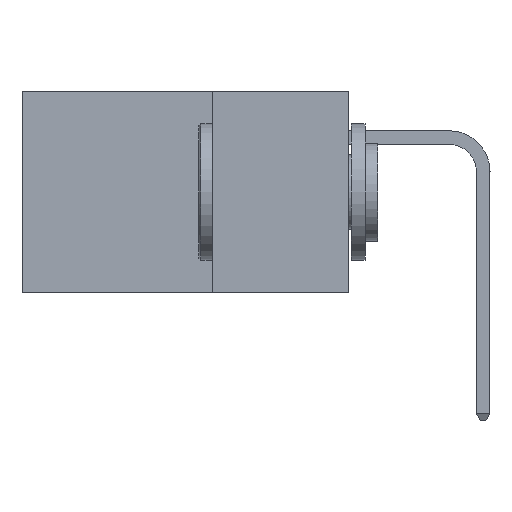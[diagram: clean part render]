
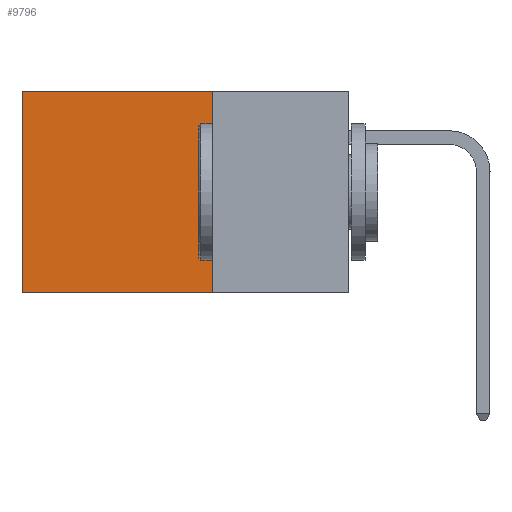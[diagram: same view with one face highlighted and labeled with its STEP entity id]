
A CAD part, left-side view. The second image highlights one B-rep face of the part: STEP entity #9796.
In plain terms, the highlighted planar face has unit normal (-1, 0, 0).
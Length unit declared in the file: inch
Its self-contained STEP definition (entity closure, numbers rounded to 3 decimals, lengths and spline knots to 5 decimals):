
#188 = CARTESIAN_POINT ( 'NONE',  ( 0.2875, 0.25, -0.37 ) ) ;
#196 = CARTESIAN_POINT ( 'NONE',  ( 0.2875, 0.25, 0. ) ) ;
#290 = CARTESIAN_POINT ( 'NONE',  ( 0.2875, 0.6, 0. ) ) ;
#325 = AXIS2_PLACEMENT_3D ( 'NONE', #196, #12470, #7125 ) ;
#1064 = EDGE_LOOP ( 'NONE', ( #6043, #9160, #12793, #15850 ) ) ;
#1556 = DIRECTION ( 'NONE',  ( 0., 0., -1. ) ) ;
#2998 = CARTESIAN_POINT ( 'NONE',  ( 0.2875, 0.25, -0.37 ) ) ;
#4681 = VECTOR ( 'NONE', #9576, 39.37008 ) ;
#5921 = VECTOR ( 'NONE', #13838, 39.37008 ) ;
#6043 = ORIENTED_EDGE ( 'NONE', *, *, #13097, .T. ) ;
#6197 = CARTESIAN_POINT ( 'NONE',  ( 0.2875, 0.25, 0. ) ) ;
#6771 = CARTESIAN_POINT ( 'NONE',  ( 0.2875, 0.6, 0. ) ) ;
#6909 = EDGE_CURVE ( 'NONE', #9263, #6946, #11709, .T. ) ;
#6946 = VERTEX_POINT ( 'NONE', #188 ) ;
#7125 = DIRECTION ( 'NONE',  ( 0., 0., -1. ) ) ;
#7304 = VECTOR ( 'NONE', #13472, 39.37008 ) ;
#7719 = EDGE_CURVE ( 'NONE', #9263, #11851, #8473, .T. ) ;
#8473 = LINE ( 'NONE', #6197, #4681 ) ;
#9160 = ORIENTED_EDGE ( 'NONE', *, *, #15967, .F. ) ;
#9263 = VERTEX_POINT ( 'NONE', #14868 ) ;
#9576 = DIRECTION ( 'NONE',  ( 0., 1., 0. ) ) ;
#9796 = ADVANCED_FACE ( 'NONE', ( #17420 ), #15151, .F. ) ;
#10397 = VERTEX_POINT ( 'NONE', #12344 ) ;
#11444 = LINE ( 'NONE', #2998, #5921 ) ;
#11709 = LINE ( 'NONE', #12343, #11918 ) ;
#11851 = VERTEX_POINT ( 'NONE', #290 ) ;
#11918 = VECTOR ( 'NONE', #1556, 39.37008 ) ;
#12343 = CARTESIAN_POINT ( 'NONE',  ( 0.2875, 0.25, 0. ) ) ;
#12344 = CARTESIAN_POINT ( 'NONE',  ( 0.2875, 0.6, -0.37 ) ) ;
#12470 = DIRECTION ( 'NONE',  ( 1., 0., 0. ) ) ;
#12793 = ORIENTED_EDGE ( 'NONE', *, *, #6909, .F. ) ;
#13097 = EDGE_CURVE ( 'NONE', #11851, #10397, #16019, .T. ) ;
#13472 = DIRECTION ( 'NONE',  ( 0., 0., -1. ) ) ;
#13838 = DIRECTION ( 'NONE',  ( 0., 1., 0. ) ) ;
#14868 = CARTESIAN_POINT ( 'NONE',  ( 0.2875, 0.25, 0. ) ) ;
#15151 = PLANE ( 'NONE',  #325 ) ;
#15850 = ORIENTED_EDGE ( 'NONE', *, *, #7719, .T. ) ;
#15967 = EDGE_CURVE ( 'NONE', #6946, #10397, #11444, .T. ) ;
#16019 = LINE ( 'NONE', #6771, #7304 ) ;
#17420 = FACE_OUTER_BOUND ( 'NONE', #1064, .T. ) ;
